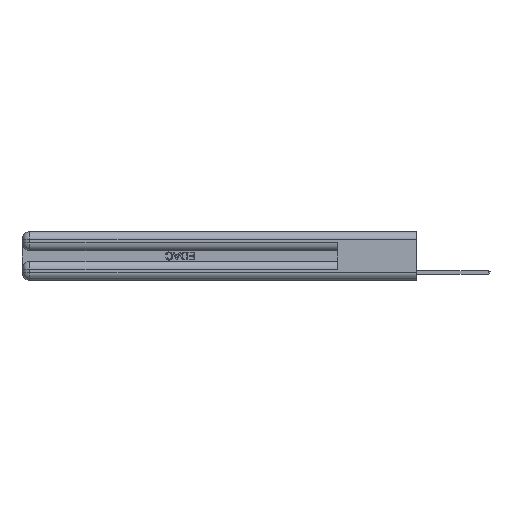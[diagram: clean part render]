
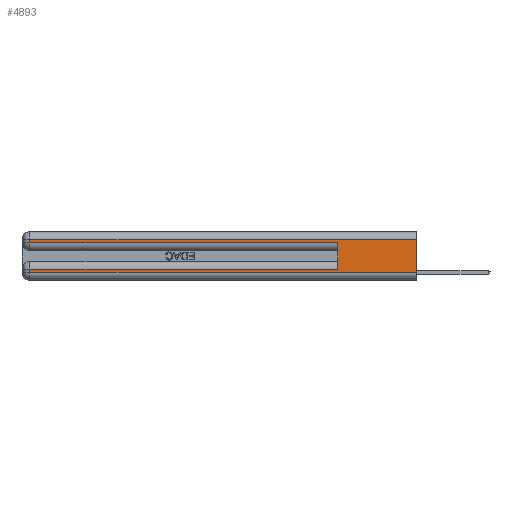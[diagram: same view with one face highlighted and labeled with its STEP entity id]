
A CAD part, left-side view. The second image highlights one B-rep face of the part: STEP entity #4893.
In plain terms, the highlighted planar face has unit normal (-1, 0, 0).
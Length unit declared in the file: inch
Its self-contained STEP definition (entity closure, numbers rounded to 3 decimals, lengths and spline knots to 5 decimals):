
#882 = DIRECTION ( 'NONE',  ( 0., 0., -1. ) ) ;
#2074 = VERTEX_POINT ( 'NONE', #30299 ) ;
#2870 = LINE ( 'NONE', #23183, #19025 ) ;
#2891 = LINE ( 'NONE', #28029, #3701 ) ;
#3463 = VERTEX_POINT ( 'NONE', #10284 ) ;
#3701 = VECTOR ( 'NONE', #22707, 39.37008 ) ;
#3794 = VECTOR ( 'NONE', #24450, 39.37008 ) ;
#4893 = ADVANCED_FACE ( 'NONE', ( #15200 ), #28277, .F. ) ;
#5032 = VERTEX_POINT ( 'NONE', #20977 ) ;
#5830 = LINE ( 'NONE', #15896, #15266 ) ;
#6473 = VECTOR ( 'NONE', #24465, 39.37008 ) ;
#6498 = EDGE_CURVE ( 'NONE', #31244, #15823, #5830, .T. ) ;
#7246 = AXIS2_PLACEMENT_3D ( 'NONE', #10575, #20649, #22631 ) ;
#7754 = CARTESIAN_POINT ( 'NONE',  ( 0., 0., 0.06 ) ) ;
#10182 = VERTEX_POINT ( 'NONE', #28100 ) ;
#10210 = VECTOR ( 'NONE', #16968, 39.37008 ) ;
#10284 = CARTESIAN_POINT ( 'NONE',  ( 0., 0.6, 0.285 ) ) ;
#10575 = CARTESIAN_POINT ( 'NONE',  ( 0., 0., 0.37 ) ) ;
#12616 = EDGE_CURVE ( 'NONE', #10182, #31244, #19325, .T. ) ;
#12867 = CARTESIAN_POINT ( 'NONE',  ( 0., 2.94, 0.285 ) ) ;
#13327 = VECTOR ( 'NONE', #29912, 39.37008 ) ;
#15188 = LINE ( 'NONE', #22292, #17337 ) ;
#15200 = FACE_OUTER_BOUND ( 'NONE', #22937, .T. ) ;
#15266 = VECTOR ( 'NONE', #28951, 39.37008 ) ;
#15460 = VERTEX_POINT ( 'NONE', #20995 ) ;
#15823 = VERTEX_POINT ( 'NONE', #7754 ) ;
#15896 = CARTESIAN_POINT ( 'NONE',  ( 0., 0., 0.06 ) ) ;
#16347 = LINE ( 'NONE', #21798, #3794 ) ;
#16808 = EDGE_CURVE ( 'NONE', #15460, #5032, #15188, .T. ) ;
#16968 = DIRECTION ( 'NONE',  ( 0., -1., 0. ) ) ;
#17034 = ORIENTED_EDGE ( 'NONE', *, *, #32059, .T. ) ;
#17131 = LINE ( 'NONE', #22072, #10210 ) ;
#17337 = VECTOR ( 'NONE', #25121, 39.37008 ) ;
#19025 = VECTOR ( 'NONE', #882, 39.37008 ) ;
#19325 = LINE ( 'NONE', #29925, #6473 ) ;
#19371 = ORIENTED_EDGE ( 'NONE', *, *, #12616, .T. ) ;
#19630 = CARTESIAN_POINT ( 'NONE',  ( 0., 0.6, 0.145 ) ) ;
#19854 = ORIENTED_EDGE ( 'NONE', *, *, #6498, .T. ) ;
#20649 = DIRECTION ( 'NONE',  ( 1., 0., 0. ) ) ;
#20977 = CARTESIAN_POINT ( 'NONE',  ( 0., 2.94, 0.31 ) ) ;
#20995 = CARTESIAN_POINT ( 'NONE',  ( 0., 0., 0.31 ) ) ;
#21798 = CARTESIAN_POINT ( 'NONE',  ( 0., 0., 0.085 ) ) ;
#21872 = CARTESIAN_POINT ( 'NONE',  ( 0., 2.94, 0.06 ) ) ;
#22072 = CARTESIAN_POINT ( 'NONE',  ( 0., 0., 0.285 ) ) ;
#22292 = CARTESIAN_POINT ( 'NONE',  ( 0., 0., 0.31 ) ) ;
#22541 = VERTEX_POINT ( 'NONE', #12867 ) ;
#22631 = DIRECTION ( 'NONE',  ( 0., 0., -1. ) ) ;
#22707 = DIRECTION ( 'NONE',  ( 0., 0., -1. ) ) ;
#22937 = EDGE_LOOP ( 'NONE', ( #31015, #31253, #30308, #32464, #27491, #17034, #19371, #19854 ) ) ;
#23183 = CARTESIAN_POINT ( 'NONE',  ( 0., 0., 0.37 ) ) ;
#23945 = EDGE_CURVE ( 'NONE', #22541, #3463, #17131, .T. ) ;
#24450 = DIRECTION ( 'NONE',  ( 0., 1., 0. ) ) ;
#24465 = DIRECTION ( 'NONE',  ( 0., 0., -1. ) ) ;
#25121 = DIRECTION ( 'NONE',  ( 0., 1., 0. ) ) ;
#27293 = EDGE_CURVE ( 'NONE', #5032, #22541, #2891, .T. ) ;
#27491 = ORIENTED_EDGE ( 'NONE', *, *, #32239, .F. ) ;
#28029 = CARTESIAN_POINT ( 'NONE',  ( 0., 2.94, 0.37 ) ) ;
#28100 = CARTESIAN_POINT ( 'NONE',  ( 0., 2.94, 0.085 ) ) ;
#28277 = PLANE ( 'NONE',  #7246 ) ;
#28951 = DIRECTION ( 'NONE',  ( 0., -1., 0. ) ) ;
#29912 = DIRECTION ( 'NONE',  ( 0., 0., 1. ) ) ;
#29925 = CARTESIAN_POINT ( 'NONE',  ( 0., 2.94, 0.37 ) ) ;
#30237 = EDGE_CURVE ( 'NONE', #15460, #15823, #2870, .T. ) ;
#30299 = CARTESIAN_POINT ( 'NONE',  ( 0., 0.6, 0.085 ) ) ;
#30308 = ORIENTED_EDGE ( 'NONE', *, *, #27293, .T. ) ;
#30407 = LINE ( 'NONE', #19630, #13327 ) ;
#31015 = ORIENTED_EDGE ( 'NONE', *, *, #30237, .F. ) ;
#31244 = VERTEX_POINT ( 'NONE', #21872 ) ;
#31253 = ORIENTED_EDGE ( 'NONE', *, *, #16808, .T. ) ;
#32059 = EDGE_CURVE ( 'NONE', #2074, #10182, #16347, .T. ) ;
#32239 = EDGE_CURVE ( 'NONE', #2074, #3463, #30407, .T. ) ;
#32464 = ORIENTED_EDGE ( 'NONE', *, *, #23945, .T. ) ;
